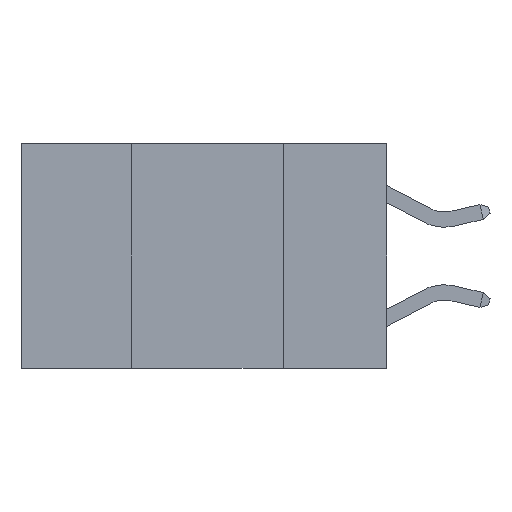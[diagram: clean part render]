
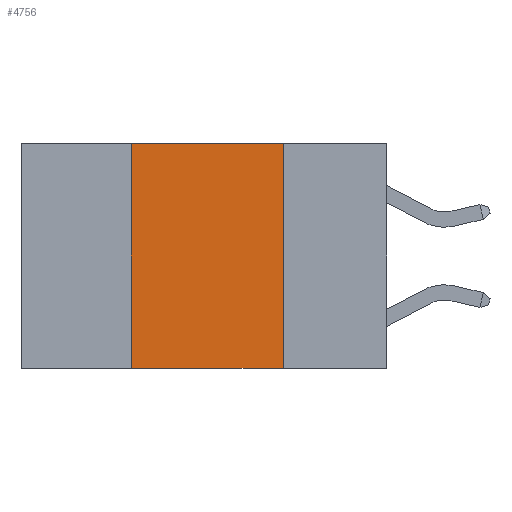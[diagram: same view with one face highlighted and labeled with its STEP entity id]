
A CAD part, left-side view. The second image highlights one B-rep face of the part: STEP entity #4756.
In plain terms, the highlighted planar face has unit normal (-1, 0, 0).
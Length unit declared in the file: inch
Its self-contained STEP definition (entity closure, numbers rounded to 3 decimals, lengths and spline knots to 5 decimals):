
#962 = LINE ( 'NONE', #2400, #18521 ) ;
#1582 = DIRECTION ( 'NONE',  ( 0., 0., -1. ) ) ;
#2400 = CARTESIAN_POINT ( 'NONE',  ( 0., 0.17, 0. ) ) ;
#3088 = CARTESIAN_POINT ( 'NONE',  ( 0., 0.42, 0. ) ) ;
#3105 = PLANE ( 'NONE',  #8302 ) ;
#3151 = VERTEX_POINT ( 'NONE', #11941 ) ;
#3721 = EDGE_LOOP ( 'NONE', ( #16739, #6341, #18939, #12218 ) ) ;
#4496 = VECTOR ( 'NONE', #11972, 39.37008 ) ;
#4756 = ADVANCED_FACE ( 'NONE', ( #18322 ), #3105, .F. ) ;
#4981 = VECTOR ( 'NONE', #17263, 39.37008 ) ;
#5094 = VERTEX_POINT ( 'NONE', #12656 ) ;
#5333 = CARTESIAN_POINT ( 'NONE',  ( 0., 0.6, -0.37 ) ) ;
#5848 = LINE ( 'NONE', #17153, #4981 ) ;
#6341 = ORIENTED_EDGE ( 'NONE', *, *, #11879, .F. ) ;
#6692 = VERTEX_POINT ( 'NONE', #18020 ) ;
#8302 = AXIS2_PLACEMENT_3D ( 'NONE', #9747, #10057, #1582 ) ;
#9297 = DIRECTION ( 'NONE',  ( 0., 0., 1. ) ) ;
#9747 = CARTESIAN_POINT ( 'NONE',  ( 0., 0.6, 0. ) ) ;
#10057 = DIRECTION ( 'NONE',  ( 1., 0., 0. ) ) ;
#10553 = DIRECTION ( 'NONE',  ( 0., 0., -1. ) ) ;
#11438 = EDGE_CURVE ( 'NONE', #13642, #3151, #962, .T. ) ;
#11879 = EDGE_CURVE ( 'NONE', #5094, #13642, #5848, .T. ) ;
#11941 = CARTESIAN_POINT ( 'NONE',  ( 0., 0.17, -0.37 ) ) ;
#11972 = DIRECTION ( 'NONE',  ( 0., -1., 0. ) ) ;
#12218 = ORIENTED_EDGE ( 'NONE', *, *, #19455, .T. ) ;
#12355 = CARTESIAN_POINT ( 'NONE',  ( 0., 0.17, 0. ) ) ;
#12489 = EDGE_CURVE ( 'NONE', #6692, #5094, #17886, .T. ) ;
#12650 = VECTOR ( 'NONE', #9297, 39.37008 ) ;
#12656 = CARTESIAN_POINT ( 'NONE',  ( 0., 0.42, 0. ) ) ;
#13642 = VERTEX_POINT ( 'NONE', #12355 ) ;
#13810 = LINE ( 'NONE', #5333, #4496 ) ;
#16739 = ORIENTED_EDGE ( 'NONE', *, *, #11438, .F. ) ;
#17153 = CARTESIAN_POINT ( 'NONE',  ( 0., 0.6, 0. ) ) ;
#17263 = DIRECTION ( 'NONE',  ( 0., -1., 0. ) ) ;
#17886 = LINE ( 'NONE', #3088, #12650 ) ;
#18020 = CARTESIAN_POINT ( 'NONE',  ( 0., 0.42, -0.37 ) ) ;
#18322 = FACE_OUTER_BOUND ( 'NONE', #3721, .T. ) ;
#18521 = VECTOR ( 'NONE', #10553, 39.37008 ) ;
#18939 = ORIENTED_EDGE ( 'NONE', *, *, #12489, .F. ) ;
#19455 = EDGE_CURVE ( 'NONE', #6692, #3151, #13810, .T. ) ;
